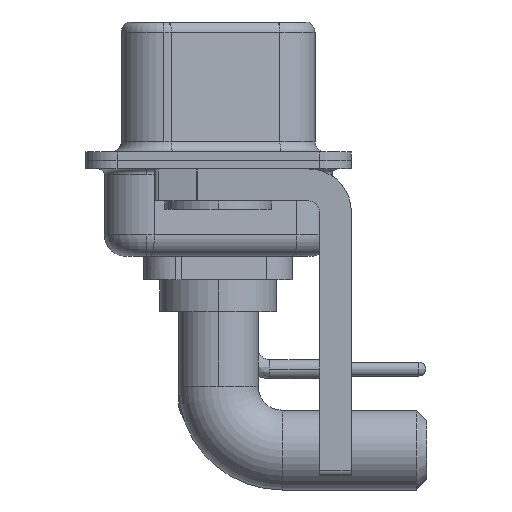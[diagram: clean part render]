
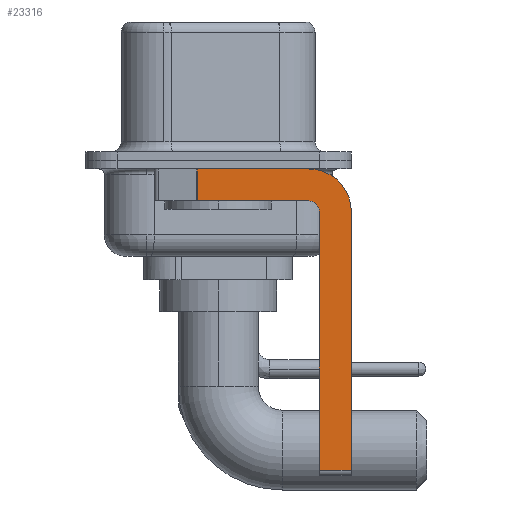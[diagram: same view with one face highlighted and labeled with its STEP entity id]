
A CAD part, left-side view. The second image highlights one B-rep face of the part: STEP entity #23316.
In plain terms, the highlighted planar face has unit normal (-1, 0, 0).
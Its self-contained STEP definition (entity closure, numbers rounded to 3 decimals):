
#167 = VECTOR ( 'NONE', #8934, 1000. ) ;
#172 = AXIS2_PLACEMENT_3D ( 'NONE', #24167, #18415, #11001 ) ;
#173 = CARTESIAN_POINT ( 'NONE',  ( -2.9, -4.25, -14.55 ) ) ;
#408 = DIRECTION ( 'NONE',  ( 0., 0., -1. ) ) ;
#448 = DIRECTION ( 'NONE',  ( -1., 0., 0. ) ) ;
#1040 = PLANE ( 'NONE',  #172 ) ;
#1245 = VERTEX_POINT ( 'NONE', #15753 ) ;
#1990 = VERTEX_POINT ( 'NONE', #6115 ) ;
#2468 = AXIS2_PLACEMENT_3D ( 'NONE', #10282, #448, #16160 ) ;
#2931 = ORIENTED_EDGE ( 'NONE', *, *, #13846, .F. ) ;
#2957 = EDGE_CURVE ( 'NONE', #23177, #1245, #19696, .T. ) ;
#5420 = CARTESIAN_POINT ( 'NONE',  ( -2.9, -6.25, -14.55 ) ) ;
#5737 = CARTESIAN_POINT ( 'NONE',  ( -2.9, 0.978, -1.9 ) ) ;
#6115 = CARTESIAN_POINT ( 'NONE',  ( -2.9, 0.978, -1.9 ) ) ;
#6187 = ORIENTED_EDGE ( 'NONE', *, *, #11198, .T. ) ;
#6271 = CARTESIAN_POINT ( 'NONE',  ( -2.9, -4.25, -2.4 ) ) ;
#7101 = CARTESIAN_POINT ( 'NONE',  ( -2.9, 0.978, -0.4 ) ) ;
#7217 = CARTESIAN_POINT ( 'NONE',  ( -2.9, -4.75, -14.55 ) ) ;
#8153 = LINE ( 'NONE', #23750, #10769 ) ;
#8934 = DIRECTION ( 'NONE',  ( 0., 1., 0. ) ) ;
#9993 = DIRECTION ( 'NONE',  ( 1., 0., 0. ) ) ;
#10282 = CARTESIAN_POINT ( 'NONE',  ( -2.9, -4.25, -2.4 ) ) ;
#10409 = VECTOR ( 'NONE', #20396, 1000. ) ;
#10769 = VECTOR ( 'NONE', #12128, 1000. ) ;
#10798 = LINE ( 'NONE', #18602, #16893 ) ;
#11001 = DIRECTION ( 'NONE',  ( 0., 0., -1. ) ) ;
#11176 = CARTESIAN_POINT ( 'NONE',  ( -2.9, 3., -0.4 ) ) ;
#11198 = EDGE_CURVE ( 'NONE', #19990, #1990, #17510, .T. ) ;
#11327 = AXIS2_PLACEMENT_3D ( 'NONE', #6271, #9993, #408 ) ;
#12128 = DIRECTION ( 'NONE',  ( 0., 0., -1. ) ) ;
#12595 = LINE ( 'NONE', #11176, #10409 ) ;
#13220 = VERTEX_POINT ( 'NONE', #20009 ) ;
#13501 = EDGE_CURVE ( 'NONE', #16038, #23177, #10798, .T. ) ;
#13846 = EDGE_CURVE ( 'NONE', #1245, #1990, #20582, .T. ) ;
#14179 = CIRCLE ( 'NONE', #11327, 2. ) ;
#14794 = EDGE_CURVE ( 'NONE', #19990, #13220, #12595, .T. ) ;
#15753 = CARTESIAN_POINT ( 'NONE',  ( -2.9, -4.25, -1.9 ) ) ;
#16038 = VERTEX_POINT ( 'NONE', #7217 ) ;
#16160 = DIRECTION ( 'NONE',  ( 0., 0., 1. ) ) ;
#16448 = EDGE_LOOP ( 'NONE', ( #24468, #6187, #2931, #24909, #21893, #24265, #19315, #19898 ) ) ;
#16893 = VECTOR ( 'NONE', #21023, 1000. ) ;
#17137 = VERTEX_POINT ( 'NONE', #20629 ) ;
#17412 = EDGE_CURVE ( 'NONE', #13220, #17137, #14179, .T. ) ;
#17510 = LINE ( 'NONE', #5737, #25054 ) ;
#17789 = CARTESIAN_POINT ( 'NONE',  ( -2.9, -4.75, -2.4 ) ) ;
#17932 = DIRECTION ( 'NONE',  ( 0., -1., 0. ) ) ;
#18002 = EDGE_CURVE ( 'NONE', #17137, #21260, #8153, .T. ) ;
#18415 = DIRECTION ( 'NONE',  ( 1., 0., 0. ) ) ;
#18602 = CARTESIAN_POINT ( 'NONE',  ( -2.9, -4.75, -14.8 ) ) ;
#19209 = VECTOR ( 'NONE', #17932, 1000. ) ;
#19315 = ORIENTED_EDGE ( 'NONE', *, *, #18002, .F. ) ;
#19696 = CIRCLE ( 'NONE', #2468, 0.5 ) ;
#19898 = ORIENTED_EDGE ( 'NONE', *, *, #17412, .F. ) ;
#19990 = VERTEX_POINT ( 'NONE', #7101 ) ;
#20009 = CARTESIAN_POINT ( 'NONE',  ( -2.9, -4.25, -0.4 ) ) ;
#20396 = DIRECTION ( 'NONE',  ( 0., -1., 0. ) ) ;
#20582 = LINE ( 'NONE', #24907, #167 ) ;
#20629 = CARTESIAN_POINT ( 'NONE',  ( -2.9, -6.25, -2.4 ) ) ;
#21023 = DIRECTION ( 'NONE',  ( 0., 0., 1. ) ) ;
#21221 = DIRECTION ( 'NONE',  ( 0., 0., -1. ) ) ;
#21260 = VERTEX_POINT ( 'NONE', #5420 ) ;
#21265 = LINE ( 'NONE', #173, #19209 ) ;
#21893 = ORIENTED_EDGE ( 'NONE', *, *, #13501, .F. ) ;
#22378 = FACE_OUTER_BOUND ( 'NONE', #16448, .T. ) ;
#23177 = VERTEX_POINT ( 'NONE', #17789 ) ;
#23316 = ADVANCED_FACE ( 'NONE', ( #22378 ), #1040, .F. ) ;
#23750 = CARTESIAN_POINT ( 'NONE',  ( -2.9, -6.25, -2.4 ) ) ;
#24167 = CARTESIAN_POINT ( 'NONE',  ( -2.9, -4.25, -2.4 ) ) ;
#24265 = ORIENTED_EDGE ( 'NONE', *, *, #24808, .T. ) ;
#24468 = ORIENTED_EDGE ( 'NONE', *, *, #14794, .F. ) ;
#24808 = EDGE_CURVE ( 'NONE', #16038, #21260, #21265, .T. ) ;
#24907 = CARTESIAN_POINT ( 'NONE',  ( -2.9, -4.25, -1.9 ) ) ;
#24909 = ORIENTED_EDGE ( 'NONE', *, *, #2957, .F. ) ;
#25054 = VECTOR ( 'NONE', #21221, 1000. ) ;
